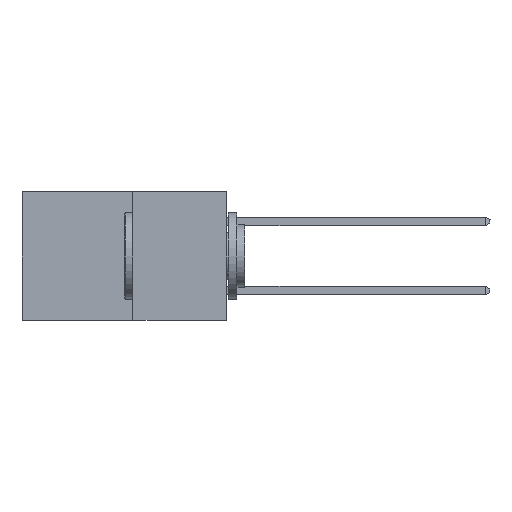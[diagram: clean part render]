
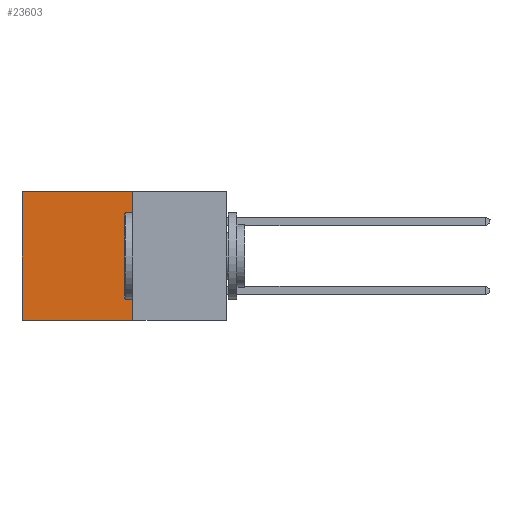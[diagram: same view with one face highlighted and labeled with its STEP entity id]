
A CAD part, left-side view. The second image highlights one B-rep face of the part: STEP entity #23603.
In plain terms, the highlighted planar face has unit normal (-1, 0, 0).
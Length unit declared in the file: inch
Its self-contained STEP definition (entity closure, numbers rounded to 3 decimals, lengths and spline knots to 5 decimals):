
#768 = VERTEX_POINT ( 'NONE', #21158 ) ;
#1549 = ORIENTED_EDGE ( 'NONE', *, *, #10498, .T. ) ;
#1677 = ORIENTED_EDGE ( 'NONE', *, *, #32530, .F. ) ;
#1911 = CARTESIAN_POINT ( 'NONE',  ( 0.277, 0.27, 0. ) ) ;
#2063 = DIRECTION ( 'NONE',  ( 0., 1., 0. ) ) ;
#5429 = CARTESIAN_POINT ( 'NONE',  ( 0.277, 0.27, -0.37 ) ) ;
#6785 = CARTESIAN_POINT ( 'NONE',  ( 0.277, 0.59, 0. ) ) ;
#6942 = CARTESIAN_POINT ( 'NONE',  ( 0.277, 0.59, -0.37 ) ) ;
#7245 = VECTOR ( 'NONE', #25751, 39.37008 ) ;
#8061 = DIRECTION ( 'NONE',  ( 0., 0., -1. ) ) ;
#9260 = EDGE_CURVE ( 'NONE', #768, #21704, #14253, .T. ) ;
#10126 = DIRECTION ( 'NONE',  ( 1., 0., 0. ) ) ;
#10498 = EDGE_CURVE ( 'NONE', #28930, #21704, #12924, .T. ) ;
#11444 = EDGE_CURVE ( 'NONE', #28334, #28930, #14390, .T. ) ;
#11707 = FACE_OUTER_BOUND ( 'NONE', #15358, .T. ) ;
#12924 = LINE ( 'NONE', #6942, #18202 ) ;
#14253 = LINE ( 'NONE', #17975, #7245 ) ;
#14390 = LINE ( 'NONE', #28008, #26500 ) ;
#15358 = EDGE_LOOP ( 'NONE', ( #1549, #30540, #1677, #23699 ) ) ;
#15977 = LINE ( 'NONE', #5429, #28093 ) ;
#17883 = CARTESIAN_POINT ( 'NONE',  ( 0.277, 0.27, -0.37 ) ) ;
#17975 = CARTESIAN_POINT ( 'NONE',  ( 0.277, 0.27, -0.37 ) ) ;
#18202 = VECTOR ( 'NONE', #32823, 39.37008 ) ;
#18899 = CARTESIAN_POINT ( 'NONE',  ( 0.277, 0.59, -0.37 ) ) ;
#21158 = CARTESIAN_POINT ( 'NONE',  ( 0.277, 0.27, -0.37 ) ) ;
#21704 = VERTEX_POINT ( 'NONE', #18899 ) ;
#23603 = ADVANCED_FACE ( 'NONE', ( #11707 ), #25663, .F. ) ;
#23699 = ORIENTED_EDGE ( 'NONE', *, *, #11444, .T. ) ;
#25663 = PLANE ( 'NONE',  #32755 ) ;
#25751 = DIRECTION ( 'NONE',  ( 0., 1., 0. ) ) ;
#26500 = VECTOR ( 'NONE', #2063, 39.37008 ) ;
#28008 = CARTESIAN_POINT ( 'NONE',  ( 0.277, 0.27, 0. ) ) ;
#28093 = VECTOR ( 'NONE', #8061, 39.37008 ) ;
#28270 = DIRECTION ( 'NONE',  ( 0., 0., -1. ) ) ;
#28334 = VERTEX_POINT ( 'NONE', #1911 ) ;
#28930 = VERTEX_POINT ( 'NONE', #6785 ) ;
#30540 = ORIENTED_EDGE ( 'NONE', *, *, #9260, .F. ) ;
#32530 = EDGE_CURVE ( 'NONE', #28334, #768, #15977, .T. ) ;
#32755 = AXIS2_PLACEMENT_3D ( 'NONE', #17883, #10126, #28270 ) ;
#32823 = DIRECTION ( 'NONE',  ( 0., 0., -1. ) ) ;
